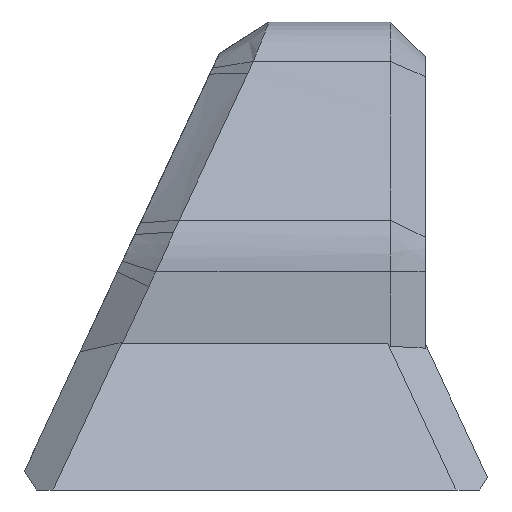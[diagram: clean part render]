
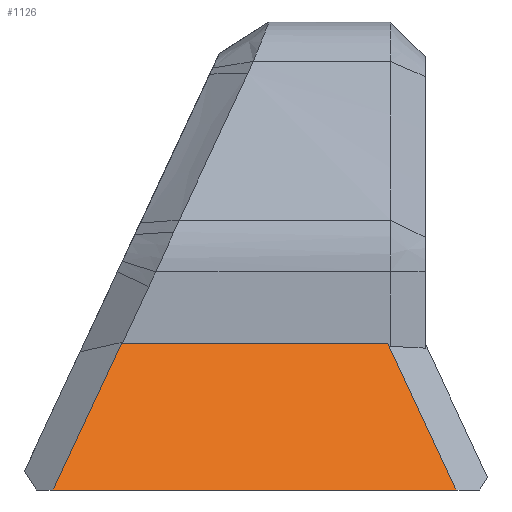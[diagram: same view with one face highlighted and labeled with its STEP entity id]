
A CAD part, left-side view. The second image highlights one B-rep face of the part: STEP entity #1126.
In plain terms, the highlighted planar face has unit normal (-0.859, 0, 0.511).
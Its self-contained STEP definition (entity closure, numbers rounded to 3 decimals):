
#148=FACE_OUTER_BOUND('',#213,.T.);
#213=EDGE_LOOP('',(#972,#973,#974,#975,#976));
#259=LINE('',#1553,#372);
#304=LINE('',#1888,#417);
#306=LINE('',#1892,#419);
#329=LINE('',#2137,#442);
#330=LINE('',#2138,#443);
#372=VECTOR('',#1297,10.);
#417=VECTOR('',#1384,10.);
#419=VECTOR('',#1388,10.);
#442=VECTOR('',#1427,10.);
#443=VECTOR('',#1428,10.);
#485=VERTEX_POINT('',#1550);
#486=VERTEX_POINT('',#1552);
#536=VERTEX_POINT('',#1882);
#538=VERTEX_POINT('',#1886);
#539=VERTEX_POINT('',#1890);
#595=EDGE_CURVE('',#485,#486,#259,.T.);
#670=EDGE_CURVE('',#538,#536,#304,.T.);
#672=EDGE_CURVE('',#539,#538,#306,.T.);
#705=EDGE_CURVE('',#536,#485,#329,.F.);
#706=EDGE_CURVE('',#539,#486,#330,.T.);
#972=ORIENTED_EDGE('',*,*,#595,.F.);
#973=ORIENTED_EDGE('',*,*,#705,.F.);
#974=ORIENTED_EDGE('',*,*,#670,.F.);
#975=ORIENTED_EDGE('',*,*,#672,.F.);
#976=ORIENTED_EDGE('',*,*,#706,.T.);
#1069=PLANE('',#1205);
#1126=ADVANCED_FACE('',(#148),#1069,.F.);
#1205=AXIS2_PLACEMENT_3D('',#2136,#1425,#1426);
#1297=DIRECTION('',(-0.475,-0.372,-0.798));
#1384=DIRECTION('',(-0.505,-0.161,-0.848));
#1388=DIRECTION('',(0.475,-0.372,0.798));
#1425=DIRECTION('center_axis',(0.859,0.,-0.511));
#1426=DIRECTION('ref_axis',(-0.511,0.,-0.859));
#1427=DIRECTION('',(0.,1.,0.));
#1428=DIRECTION('',(0.,-1.,0.));
#1550=CARTESIAN_POINT('',(-9.5,1.078,2.1));
#1552=CARTESIAN_POINT('',(-10.75,0.097,0.));
#1553=CARTESIAN_POINT('',(-10.704,0.133,0.077));
#1882=CARTESIAN_POINT('',(-9.5,4.888,2.1));
#1886=CARTESIAN_POINT('',(-9.488,4.892,2.12));
#1888=CARTESIAN_POINT('',(-9.347,4.937,2.358));
#1890=CARTESIAN_POINT('',(-10.75,5.881,0.));
#1892=CARTESIAN_POINT('',(-8.711,4.282,3.426));
#2136=CARTESIAN_POINT('Origin',(-9.5,-5.38,2.1));
#2137=CARTESIAN_POINT('',(-9.5,-0.04,2.1));
#2138=CARTESIAN_POINT('',(-10.75,6.42,0.));
